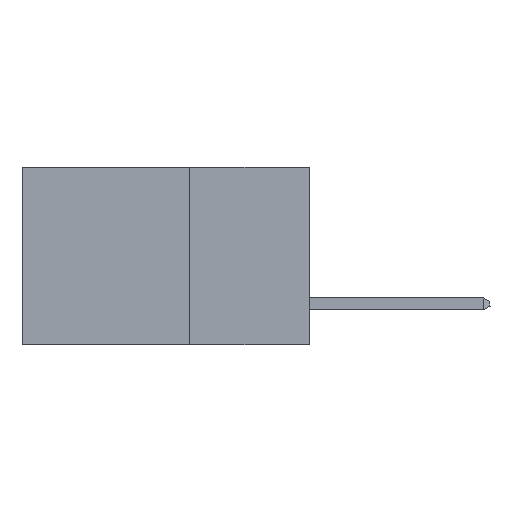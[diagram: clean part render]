
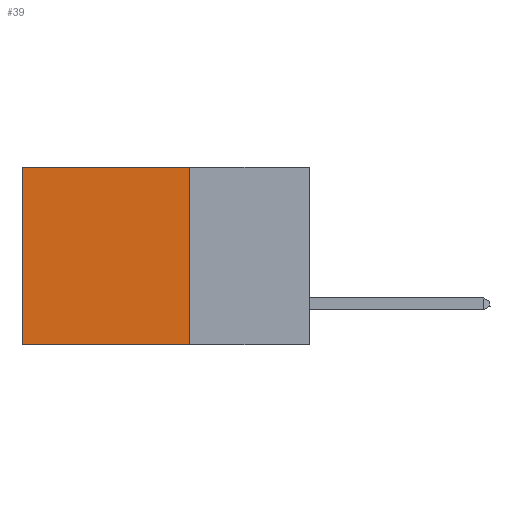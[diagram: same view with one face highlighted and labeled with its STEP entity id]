
A CAD part, left-side view. The second image highlights one B-rep face of the part: STEP entity #39.
In plain terms, the highlighted planar face has unit normal (-1, 0, 0).
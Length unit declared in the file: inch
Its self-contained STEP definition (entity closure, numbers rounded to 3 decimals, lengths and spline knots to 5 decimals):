
#16 = FACE_OUTER_BOUND ( 'NONE', #5440, .T. ) ;
#39 = ADVANCED_FACE ( 'NONE', ( #16 ), #3689, .F. ) ;
#1298 = DIRECTION ( 'NONE',  ( 0., 1., 0. ) ) ;
#1440 = ORIENTED_EDGE ( 'NONE', *, *, #11111, .F. ) ;
#1799 = CARTESIAN_POINT ( 'NONE',  ( 0.2875, 0.25, 0. ) ) ;
#1947 = LINE ( 'NONE', #8454, #8554 ) ;
#1950 = CARTESIAN_POINT ( 'NONE',  ( 0.2875, 0.25, 0. ) ) ;
#2091 = VECTOR ( 'NONE', #5226, 39.37008 ) ;
#2639 = VERTEX_POINT ( 'NONE', #1799 ) ;
#2911 = VERTEX_POINT ( 'NONE', #7021 ) ;
#3200 = CARTESIAN_POINT ( 'NONE',  ( 0.2875, 0.6, 0. ) ) ;
#3629 = ORIENTED_EDGE ( 'NONE', *, *, #9263, .T. ) ;
#3689 = PLANE ( 'NONE',  #8890 ) ;
#3804 = ORIENTED_EDGE ( 'NONE', *, *, #6162, .T. ) ;
#4716 = DIRECTION ( 'NONE',  ( 0., 0., -1. ) ) ;
#4724 = VERTEX_POINT ( 'NONE', #5256 ) ;
#4947 = DIRECTION ( 'NONE',  ( 0., 0., -1. ) ) ;
#5226 = DIRECTION ( 'NONE',  ( 0., 0., -1. ) ) ;
#5256 = CARTESIAN_POINT ( 'NONE',  ( 0.2875, 0.6, 0. ) ) ;
#5440 = EDGE_LOOP ( 'NONE', ( #3804, #7572, #1440, #3629 ) ) ;
#5443 = VECTOR ( 'NONE', #4947, 39.37008 ) ;
#5521 = EDGE_CURVE ( 'NONE', #7427, #2911, #1947, .T. ) ;
#5753 = LINE ( 'NONE', #9959, #5443 ) ;
#6162 = EDGE_CURVE ( 'NONE', #4724, #2911, #8060, .T. ) ;
#7021 = CARTESIAN_POINT ( 'NONE',  ( 0.2875, 0.6, -0.37 ) ) ;
#7378 = VECTOR ( 'NONE', #8990, 39.37008 ) ;
#7427 = VERTEX_POINT ( 'NONE', #11686 ) ;
#7572 = ORIENTED_EDGE ( 'NONE', *, *, #5521, .F. ) ;
#8060 = LINE ( 'NONE', #3200, #2091 ) ;
#8454 = CARTESIAN_POINT ( 'NONE',  ( 0.2875, 0.25, -0.37 ) ) ;
#8554 = VECTOR ( 'NONE', #1298, 39.37008 ) ;
#8743 = CARTESIAN_POINT ( 'NONE',  ( 0.2875, 0.25, 0. ) ) ;
#8890 = AXIS2_PLACEMENT_3D ( 'NONE', #8743, #10771, #4716 ) ;
#8990 = DIRECTION ( 'NONE',  ( 0., 1., 0. ) ) ;
#9263 = EDGE_CURVE ( 'NONE', #2639, #4724, #11498, .T. ) ;
#9959 = CARTESIAN_POINT ( 'NONE',  ( 0.2875, 0.25, 0. ) ) ;
#10771 = DIRECTION ( 'NONE',  ( 1., 0., 0. ) ) ;
#11111 = EDGE_CURVE ( 'NONE', #2639, #7427, #5753, .T. ) ;
#11498 = LINE ( 'NONE', #1950, #7378 ) ;
#11686 = CARTESIAN_POINT ( 'NONE',  ( 0.2875, 0.25, -0.37 ) ) ;
